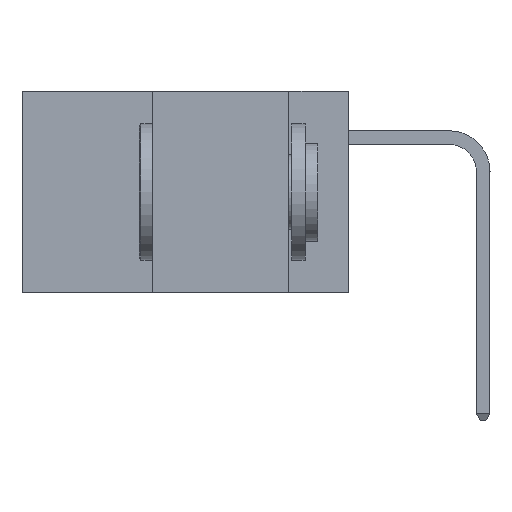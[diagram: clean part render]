
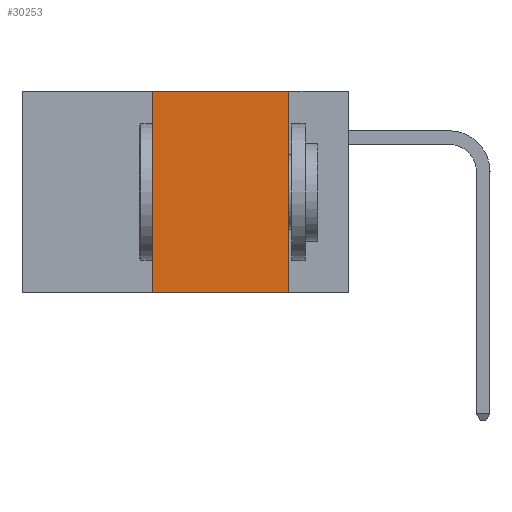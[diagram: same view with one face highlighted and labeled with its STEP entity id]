
A CAD part, left-side view. The second image highlights one B-rep face of the part: STEP entity #30253.
In plain terms, the highlighted planar face has unit normal (-1, 0, 0).
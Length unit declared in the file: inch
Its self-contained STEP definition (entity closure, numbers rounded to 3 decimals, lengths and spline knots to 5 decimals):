
#98 = AXIS2_PLACEMENT_3D ( 'NONE', #30335, #37063, #18688 ) ;
#2065 = VECTOR ( 'NONE', #25430, 39.37008 ) ;
#2278 = VERTEX_POINT ( 'NONE', #42625 ) ;
#3604 = DIRECTION ( 'NONE',  ( 0., -1., 0. ) ) ;
#6021 = CARTESIAN_POINT ( 'NONE',  ( 0., 0.11, 0. ) ) ;
#8851 = FACE_OUTER_BOUND ( 'NONE', #30913, .T. ) ;
#9479 = VERTEX_POINT ( 'NONE', #28690 ) ;
#9489 = VECTOR ( 'NONE', #25573, 39.37008 ) ;
#15081 = PLANE ( 'NONE',  #98 ) ;
#17259 = VECTOR ( 'NONE', #39762, 39.37008 ) ;
#17379 = EDGE_CURVE ( 'NONE', #2278, #9479, #20206, .T. ) ;
#18688 = DIRECTION ( 'NONE',  ( 0., 0., -1. ) ) ;
#19007 = LINE ( 'NONE', #48456, #43020 ) ;
#20206 = LINE ( 'NONE', #40672, #2065 ) ;
#21669 = EDGE_CURVE ( 'NONE', #9479, #33578, #19007, .T. ) ;
#24222 = CARTESIAN_POINT ( 'NONE',  ( 0., 0.11, -0.37 ) ) ;
#25085 = CARTESIAN_POINT ( 'NONE',  ( 0., 0.6, -0.37 ) ) ;
#25430 = DIRECTION ( 'NONE',  ( 0., 0., 1. ) ) ;
#25573 = DIRECTION ( 'NONE',  ( 0., -1., 0. ) ) ;
#26744 = ORIENTED_EDGE ( 'NONE', *, *, #17379, .F. ) ;
#28690 = CARTESIAN_POINT ( 'NONE',  ( 0., 0.36, 0. ) ) ;
#29462 = LINE ( 'NONE', #25085, #9489 ) ;
#30037 = EDGE_CURVE ( 'NONE', #2278, #43319, #29462, .T. ) ;
#30253 = ADVANCED_FACE ( 'NONE', ( #8851 ), #15081, .F. ) ;
#30335 = CARTESIAN_POINT ( 'NONE',  ( 0., 0.6, 0. ) ) ;
#30913 = EDGE_LOOP ( 'NONE', ( #46444, #46644, #26744, #46141 ) ) ;
#33578 = VERTEX_POINT ( 'NONE', #34025 ) ;
#34025 = CARTESIAN_POINT ( 'NONE',  ( 0., 0.11, 0. ) ) ;
#36754 = EDGE_CURVE ( 'NONE', #33578, #43319, #37981, .T. ) ;
#37063 = DIRECTION ( 'NONE',  ( 1., 0., 0. ) ) ;
#37981 = LINE ( 'NONE', #6021, #17259 ) ;
#39762 = DIRECTION ( 'NONE',  ( 0., 0., -1. ) ) ;
#40672 = CARTESIAN_POINT ( 'NONE',  ( 0., 0.36, 0. ) ) ;
#42625 = CARTESIAN_POINT ( 'NONE',  ( 0., 0.36, -0.37 ) ) ;
#43020 = VECTOR ( 'NONE', #3604, 39.37008 ) ;
#43319 = VERTEX_POINT ( 'NONE', #24222 ) ;
#46141 = ORIENTED_EDGE ( 'NONE', *, *, #30037, .T. ) ;
#46444 = ORIENTED_EDGE ( 'NONE', *, *, #36754, .F. ) ;
#46644 = ORIENTED_EDGE ( 'NONE', *, *, #21669, .F. ) ;
#48456 = CARTESIAN_POINT ( 'NONE',  ( 0., 0.6, 0. ) ) ;
